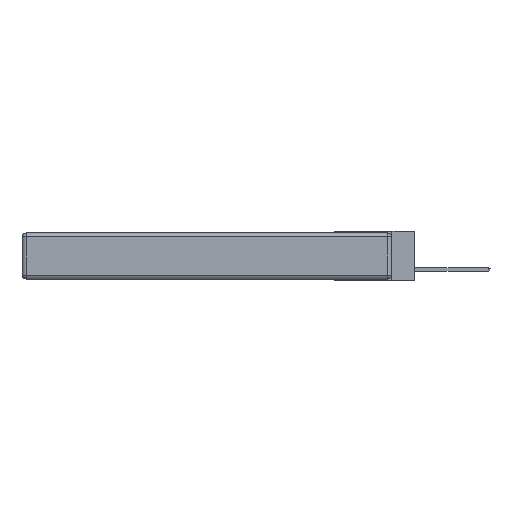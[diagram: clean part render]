
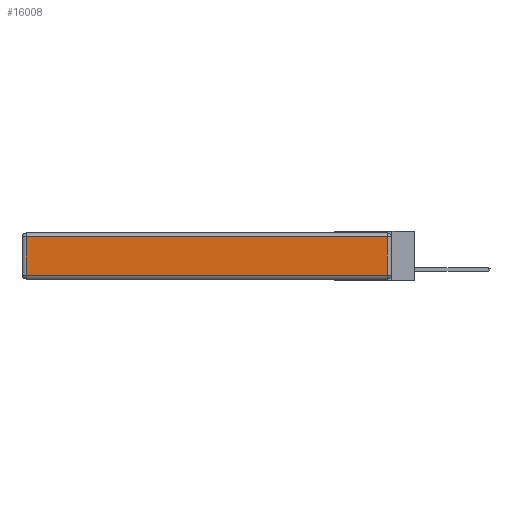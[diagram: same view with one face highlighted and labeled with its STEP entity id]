
A CAD part, left-side view. The second image highlights one B-rep face of the part: STEP entity #16008.
In plain terms, the highlighted planar face has unit normal (-1, 0, 0).
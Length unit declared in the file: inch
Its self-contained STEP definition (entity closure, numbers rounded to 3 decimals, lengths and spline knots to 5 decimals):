
#919 = DIRECTION ( 'NONE',  ( 0., 1., 0. ) ) ;
#962 = CARTESIAN_POINT ( 'NONE',  ( 0., 0., -0.313 ) ) ;
#994 = VERTEX_POINT ( 'NONE', #1891 ) ;
#1103 = ORIENTED_EDGE ( 'NONE', *, *, #2905, .T. ) ;
#1891 = CARTESIAN_POINT ( 'NONE',  ( 0., 0.03, -0.313 ) ) ;
#2905 = EDGE_CURVE ( 'NONE', #4034, #2994, #3676, .T. ) ;
#2994 = VERTEX_POINT ( 'NONE', #19474 ) ;
#3676 = LINE ( 'NONE', #5285, #22035 ) ;
#4034 = VERTEX_POINT ( 'NONE', #17232 ) ;
#4127 = DIRECTION ( 'NONE',  ( 0., 0., 1. ) ) ;
#4182 = FACE_OUTER_BOUND ( 'NONE', #18676, .T. ) ;
#4297 = CARTESIAN_POINT ( 'NONE',  ( 0., 2.75, -0.03 ) ) ;
#4482 = AXIS2_PLACEMENT_3D ( 'NONE', #8958, #5571, #16259 ) ;
#4738 = VECTOR ( 'NONE', #10127, 39.37008 ) ;
#5285 = CARTESIAN_POINT ( 'NONE',  ( 0., 2.72, -0.343 ) ) ;
#5571 = DIRECTION ( 'NONE',  ( -1., 0., 0. ) ) ;
#6042 = VERTEX_POINT ( 'NONE', #7818 ) ;
#6182 = ORIENTED_EDGE ( 'NONE', *, *, #18693, .T. ) ;
#7479 = VECTOR ( 'NONE', #919, 39.37008 ) ;
#7818 = CARTESIAN_POINT ( 'NONE',  ( 0., 0.03, -0.03 ) ) ;
#7929 = ORIENTED_EDGE ( 'NONE', *, *, #13482, .T. ) ;
#8109 = LINE ( 'NONE', #14689, #16516 ) ;
#8958 = CARTESIAN_POINT ( 'NONE',  ( 0., 0., -0.343 ) ) ;
#10127 = DIRECTION ( 'NONE',  ( 0., -1., 0. ) ) ;
#10320 = DIRECTION ( 'NONE',  ( 0., 0., -1. ) ) ;
#10706 = ORIENTED_EDGE ( 'NONE', *, *, #14887, .T. ) ;
#10843 = PLANE ( 'NONE',  #4482 ) ;
#11664 = LINE ( 'NONE', #4297, #7479 ) ;
#13482 = EDGE_CURVE ( 'NONE', #994, #6042, #8109, .T. ) ;
#14689 = CARTESIAN_POINT ( 'NONE',  ( 0., 0.03, -0.343 ) ) ;
#14887 = EDGE_CURVE ( 'NONE', #6042, #4034, #11664, .T. ) ;
#15044 = LINE ( 'NONE', #962, #4738 ) ;
#16008 = ADVANCED_FACE ( 'NONE', ( #4182 ), #10843, .T. ) ;
#16259 = DIRECTION ( 'NONE',  ( 0., 0., 1. ) ) ;
#16516 = VECTOR ( 'NONE', #4127, 39.37008 ) ;
#17232 = CARTESIAN_POINT ( 'NONE',  ( 0., 2.72, -0.03 ) ) ;
#18676 = EDGE_LOOP ( 'NONE', ( #6182, #7929, #10706, #1103 ) ) ;
#18693 = EDGE_CURVE ( 'NONE', #2994, #994, #15044, .T. ) ;
#19474 = CARTESIAN_POINT ( 'NONE',  ( 0., 2.72, -0.313 ) ) ;
#22035 = VECTOR ( 'NONE', #10320, 39.37008 ) ;
